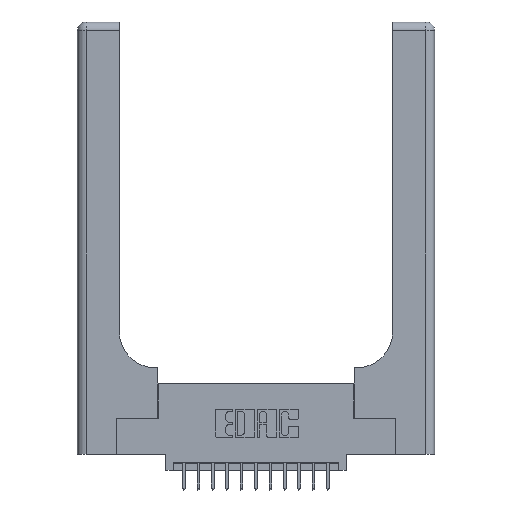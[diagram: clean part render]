
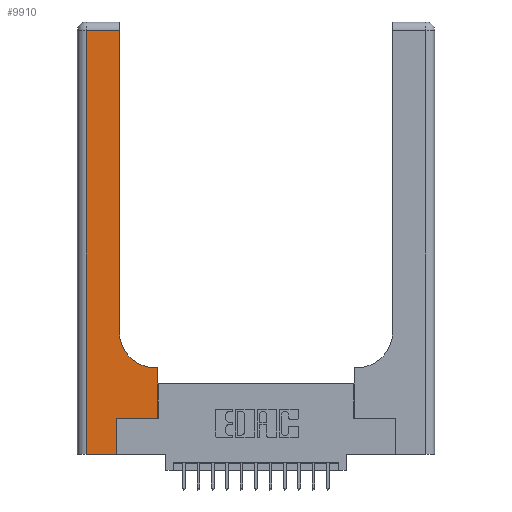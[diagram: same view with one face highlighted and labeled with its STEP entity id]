
A CAD part, top view. The second image highlights one B-rep face of the part: STEP entity #9910.
In plain terms, the highlighted planar face has unit normal (0, 0, 1).
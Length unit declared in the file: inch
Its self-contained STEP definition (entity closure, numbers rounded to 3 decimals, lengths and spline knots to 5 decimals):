
#165 = EDGE_CURVE ( 'NONE', #6923, #10098, #10369, .T. ) ;
#875 = DIRECTION ( 'NONE',  ( -1., 0., 0. ) ) ;
#966 = EDGE_CURVE ( 'NONE', #9063, #14522, #10390, .T. ) ;
#1362 = EDGE_CURVE ( 'NONE', #2420, #14751, #7347, .T. ) ;
#1374 = VECTOR ( 'NONE', #6247, 39.37008 ) ;
#1376 = DIRECTION ( 'NONE',  ( 1., 0., 0. ) ) ;
#1630 = VECTOR ( 'NONE', #11526, 39.37008 ) ;
#2055 = LINE ( 'NONE', #7450, #1630 ) ;
#2078 = VERTEX_POINT ( 'NONE', #3208 ) ;
#2420 = VERTEX_POINT ( 'NONE', #13289 ) ;
#2511 = LINE ( 'NONE', #14229, #14519 ) ;
#2581 = ORIENTED_EDGE ( 'NONE', *, *, #13098, .T. ) ;
#3167 = CARTESIAN_POINT ( 'NONE',  ( 0.5585, 0.25, 0.37 ) ) ;
#3208 = CARTESIAN_POINT ( 'NONE',  ( 0.06, 0., 0.37 ) ) ;
#3273 = ORIENTED_EDGE ( 'NONE', *, *, #4088, .T. ) ;
#3371 = DIRECTION ( 'NONE',  ( 0., -1., 0. ) ) ;
#3846 = ORIENTED_EDGE ( 'NONE', *, *, #4984, .T. ) ;
#3852 = VECTOR ( 'NONE', #17271, 39.37008 ) ;
#3976 = EDGE_CURVE ( 'NONE', #2078, #2420, #8225, .T. ) ;
#4088 = EDGE_CURVE ( 'NONE', #11182, #14825, #10356, .T. ) ;
#4150 = CARTESIAN_POINT ( 'NONE',  ( 0., 0., 0.37 ) ) ;
#4286 = CARTESIAN_POINT ( 'NONE',  ( 0.5415, 0.6, 0.37 ) ) ;
#4582 = CARTESIAN_POINT ( 'NONE',  ( 0.5585, 0.25, 0.37 ) ) ;
#4826 = LINE ( 'NONE', #14625, #12342 ) ;
#4984 = EDGE_CURVE ( 'NONE', #14825, #2078, #4826, .T. ) ;
#5589 = ORIENTED_EDGE ( 'NONE', *, *, #3976, .T. ) ;
#5618 = DIRECTION ( 'NONE',  ( 1., 0., 0. ) ) ;
#5734 = DIRECTION ( 'NONE',  ( 0., 0., -1. ) ) ;
#5889 = CARTESIAN_POINT ( 'NONE',  ( 0., 2.94, 0.37 ) ) ;
#6247 = DIRECTION ( 'NONE',  ( -1., 0., 0. ) ) ;
#6737 = CARTESIAN_POINT ( 'NONE',  ( 0.06, 2.94, 0.37 ) ) ;
#6865 = PLANE ( 'NONE',  #13127 ) ;
#6923 = VERTEX_POINT ( 'NONE', #4286 ) ;
#6935 = DIRECTION ( 'NONE',  ( 0., 1., 0. ) ) ;
#7347 = LINE ( 'NONE', #15835, #7982 ) ;
#7450 = CARTESIAN_POINT ( 'NONE',  ( 0.2915, 0.6, 0.37 ) ) ;
#7904 = FACE_OUTER_BOUND ( 'NONE', #17318, .T. ) ;
#7982 = VECTOR ( 'NONE', #6935, 39.37008 ) ;
#7984 = AXIS2_PLACEMENT_3D ( 'NONE', #15614, #5734, #1376 ) ;
#7989 = DIRECTION ( 'NONE',  ( 0., 0., -1. ) ) ;
#8225 = LINE ( 'NONE', #4150, #12600 ) ;
#9014 = EDGE_CURVE ( 'NONE', #14522, #6923, #2055, .T. ) ;
#9063 = VERTEX_POINT ( 'NONE', #4582 ) ;
#9298 = CARTESIAN_POINT ( 'NONE',  ( 0., 3., 0.37 ) ) ;
#9365 = ORIENTED_EDGE ( 'NONE', *, *, #165, .T. ) ;
#9910 = ADVANCED_FACE ( 'NONE', ( #7904 ), #6865, .F. ) ;
#9938 = ORIENTED_EDGE ( 'NONE', *, *, #14433, .T. ) ;
#9952 = CARTESIAN_POINT ( 'NONE',  ( 0.2915, 2.94, 0.37 ) ) ;
#10098 = VERTEX_POINT ( 'NONE', #12922 ) ;
#10356 = LINE ( 'NONE', #5889, #1374 ) ;
#10369 = CIRCLE ( 'NONE', #7984, 0.25 ) ;
#10390 = LINE ( 'NONE', #3167, #3852 ) ;
#10443 = LINE ( 'NONE', #11626, #15738 ) ;
#10739 = ORIENTED_EDGE ( 'NONE', *, *, #1362, .T. ) ;
#11182 = VERTEX_POINT ( 'NONE', #9952 ) ;
#11513 = CARTESIAN_POINT ( 'NONE',  ( 0.5585, 0.6, 0.37 ) ) ;
#11526 = DIRECTION ( 'NONE',  ( -1., 0., 0. ) ) ;
#11626 = CARTESIAN_POINT ( 'NONE',  ( 0.2915, 3., 0.37 ) ) ;
#11732 = DIRECTION ( 'NONE',  ( 1., 0., 0. ) ) ;
#12342 = VECTOR ( 'NONE', #3371, 39.37008 ) ;
#12600 = VECTOR ( 'NONE', #5618, 39.37008 ) ;
#12922 = CARTESIAN_POINT ( 'NONE',  ( 0.2915, 0.85, 0.37 ) ) ;
#13098 = EDGE_CURVE ( 'NONE', #14751, #9063, #2511, .T. ) ;
#13127 = AXIS2_PLACEMENT_3D ( 'NONE', #9298, #7989, #875 ) ;
#13289 = CARTESIAN_POINT ( 'NONE',  ( 0.269, 0., 0.37 ) ) ;
#14229 = CARTESIAN_POINT ( 'NONE',  ( 0.269, 0.25, 0.37 ) ) ;
#14433 = EDGE_CURVE ( 'NONE', #10098, #11182, #10443, .T. ) ;
#14519 = VECTOR ( 'NONE', #11732, 39.37008 ) ;
#14522 = VERTEX_POINT ( 'NONE', #11513 ) ;
#14625 = CARTESIAN_POINT ( 'NONE',  ( 0.06, 3., 0.37 ) ) ;
#14751 = VERTEX_POINT ( 'NONE', #15908 ) ;
#14825 = VERTEX_POINT ( 'NONE', #6737 ) ;
#15521 = ORIENTED_EDGE ( 'NONE', *, *, #966, .T. ) ;
#15614 = CARTESIAN_POINT ( 'NONE',  ( 0.5415, 0.85, 0.37 ) ) ;
#15738 = VECTOR ( 'NONE', #16018, 39.37008 ) ;
#15835 = CARTESIAN_POINT ( 'NONE',  ( 0.269, 0., 0.37 ) ) ;
#15908 = CARTESIAN_POINT ( 'NONE',  ( 0.269, 0.25, 0.37 ) ) ;
#16018 = DIRECTION ( 'NONE',  ( 0., 1., 0. ) ) ;
#17124 = ORIENTED_EDGE ( 'NONE', *, *, #9014, .T. ) ;
#17271 = DIRECTION ( 'NONE',  ( 0., 1., 0. ) ) ;
#17318 = EDGE_LOOP ( 'NONE', ( #9938, #3273, #3846, #5589, #10739, #2581, #15521, #17124, #9365 ) ) ;
